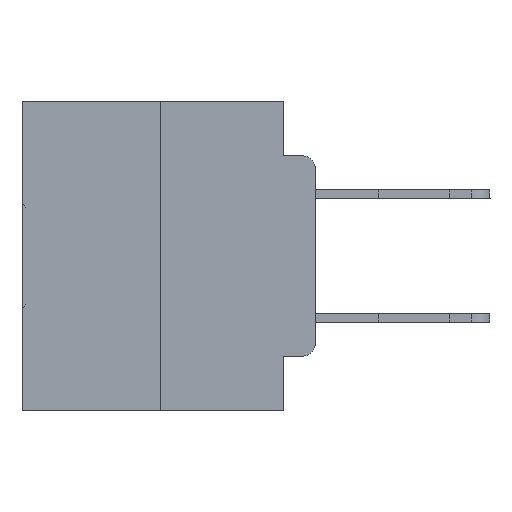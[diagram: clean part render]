
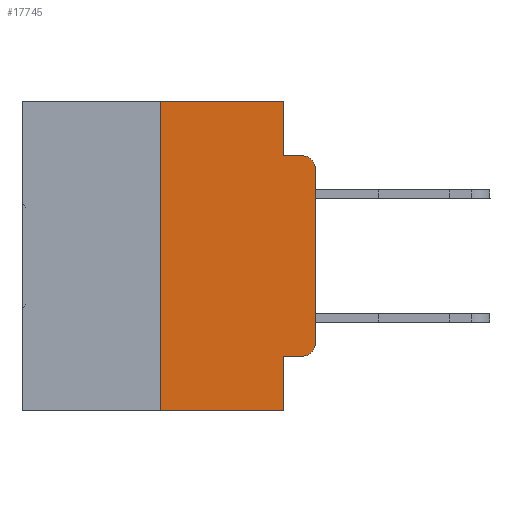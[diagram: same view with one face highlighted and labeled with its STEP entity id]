
A CAD part, left-side view. The second image highlights one B-rep face of the part: STEP entity #17745.
In plain terms, the highlighted planar face has unit normal (-1, 0, 0).
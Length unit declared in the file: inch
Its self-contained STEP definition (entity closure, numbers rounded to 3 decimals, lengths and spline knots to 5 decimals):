
#335 = ORIENTED_EDGE ( 'NONE', *, *, #4271, .F. ) ;
#445 = VECTOR ( 'NONE', #6313, 39.37008 ) ;
#823 = EDGE_CURVE ( 'NONE', #12405, #17345, #31965, .T. ) ;
#1919 = CIRCLE ( 'NONE', #31262, 0.02 ) ;
#2372 = ORIENTED_EDGE ( 'NONE', *, *, #3006, .T. ) ;
#2448 = AXIS2_PLACEMENT_3D ( 'NONE', #12802, #29903, #15337 ) ;
#2671 = ORIENTED_EDGE ( 'NONE', *, *, #28006, .F. ) ;
#3006 = EDGE_CURVE ( 'NONE', #11689, #9066, #28833, .T. ) ;
#3273 = CARTESIAN_POINT ( 'NONE',  ( 0., 0.051, 0. ) ) ;
#3551 = VECTOR ( 'NONE', #8623, 39.37008 ) ;
#3740 = CARTESIAN_POINT ( 'NONE',  ( 0., 0., 0. ) ) ;
#4138 = VERTEX_POINT ( 'NONE', #29300 ) ;
#4271 = EDGE_CURVE ( 'NONE', #17345, #9781, #13915, .T. ) ;
#4368 = ORIENTED_EDGE ( 'NONE', *, *, #29582, .F. ) ;
#5059 = CARTESIAN_POINT ( 'NONE',  ( 0., 0.051, -0.4115 ) ) ;
#6313 = DIRECTION ( 'NONE',  ( 0., 0., 1. ) ) ;
#6607 = DIRECTION ( 'NONE',  ( -1., 0., 0. ) ) ;
#7069 = CARTESIAN_POINT ( 'NONE',  ( 0., 0.473, 0. ) ) ;
#7554 = CARTESIAN_POINT ( 'NONE',  ( 0., 0.051, -0.4115 ) ) ;
#7565 = VECTOR ( 'NONE', #21828, 39.37008 ) ;
#7703 = EDGE_CURVE ( 'NONE', #4138, #9781, #1919, .T. ) ;
#8623 = DIRECTION ( 'NONE',  ( 0., 0., 1. ) ) ;
#9066 = VERTEX_POINT ( 'NONE', #27951 ) ;
#9092 = DIRECTION ( 'NONE',  ( -1., 0., 0. ) ) ;
#9589 = AXIS2_PLACEMENT_3D ( 'NONE', #23738, #9092, #26189 ) ;
#9726 = FACE_OUTER_BOUND ( 'NONE', #14275, .T. ) ;
#9781 = VERTEX_POINT ( 'NONE', #20885 ) ;
#9907 = LINE ( 'NONE', #7069, #22913 ) ;
#10166 = VECTOR ( 'NONE', #16653, 39.37008 ) ;
#11091 = EDGE_CURVE ( 'NONE', #13389, #4138, #13869, .T. ) ;
#11689 = VERTEX_POINT ( 'NONE', #30651 ) ;
#12196 = VECTOR ( 'NONE', #19856, 39.37008 ) ;
#12405 = VERTEX_POINT ( 'NONE', #23756 ) ;
#12802 = CARTESIAN_POINT ( 'NONE',  ( 0., 0.473, 0. ) ) ;
#13111 = VECTOR ( 'NONE', #23097, 39.37008 ) ;
#13389 = VERTEX_POINT ( 'NONE', #23079 ) ;
#13607 = CARTESIAN_POINT ( 'NONE',  ( 0., 0.25, 0. ) ) ;
#13869 = LINE ( 'NONE', #3740, #445 ) ;
#13915 = LINE ( 'NONE', #24008, #14637 ) ;
#14085 = VERTEX_POINT ( 'NONE', #20551 ) ;
#14275 = EDGE_LOOP ( 'NONE', ( #21618, #28159, #335, #15859, #25833, #4368, #2372, #2671, #26941, #21997 ) ) ;
#14637 = VECTOR ( 'NONE', #24073, 39.37008 ) ;
#15337 = DIRECTION ( 'NONE',  ( 0., 0., -1. ) ) ;
#15859 = ORIENTED_EDGE ( 'NONE', *, *, #823, .F. ) ;
#16653 = DIRECTION ( 'NONE',  ( 0., -1., 0. ) ) ;
#16803 = LINE ( 'NONE', #13607, #3551 ) ;
#17345 = VERTEX_POINT ( 'NONE', #18698 ) ;
#17745 = ADVANCED_FACE ( 'NONE', ( #9726 ), #22616, .F. ) ;
#18312 = VERTEX_POINT ( 'NONE', #7554 ) ;
#18698 = CARTESIAN_POINT ( 'NONE',  ( 0., 0.051, -0.0885 ) ) ;
#19856 = DIRECTION ( 'NONE',  ( 0., -1., 0. ) ) ;
#20377 = CARTESIAN_POINT ( 'NONE',  ( 0., 0.473, -0.5 ) ) ;
#20551 = CARTESIAN_POINT ( 'NONE',  ( 0., 0.02, -0.4115 ) ) ;
#20885 = CARTESIAN_POINT ( 'NONE',  ( 0., 0.02, -0.0885 ) ) ;
#21351 = CARTESIAN_POINT ( 'NONE',  ( 0., 0.02, -0.1085 ) ) ;
#21484 = EDGE_CURVE ( 'NONE', #14085, #13389, #31944, .T. ) ;
#21618 = ORIENTED_EDGE ( 'NONE', *, *, #11091, .T. ) ;
#21795 = CARTESIAN_POINT ( 'NONE',  ( 0., 0.051, 0. ) ) ;
#21828 = DIRECTION ( 'NONE',  ( 0., 0., -1. ) ) ;
#21997 = ORIENTED_EDGE ( 'NONE', *, *, #21484, .T. ) ;
#22616 = PLANE ( 'NONE',  #2448 ) ;
#22913 = VECTOR ( 'NONE', #24222, 39.37008 ) ;
#23079 = CARTESIAN_POINT ( 'NONE',  ( 0., 0., -0.3915 ) ) ;
#23097 = DIRECTION ( 'NONE',  ( 0., 0., -1. ) ) ;
#23738 = CARTESIAN_POINT ( 'NONE',  ( 0., 0.02, -0.3915 ) ) ;
#23756 = CARTESIAN_POINT ( 'NONE',  ( 0., 0.051, 0. ) ) ;
#23796 = DIRECTION ( 'NONE',  ( 0., 0., -1. ) ) ;
#24008 = CARTESIAN_POINT ( 'NONE',  ( 0., 0.051, -0.0885 ) ) ;
#24073 = DIRECTION ( 'NONE',  ( 0., -1., 0. ) ) ;
#24222 = DIRECTION ( 'NONE',  ( 0., -1., 0. ) ) ;
#24729 = EDGE_CURVE ( 'NONE', #18312, #14085, #25165, .T. ) ;
#25165 = LINE ( 'NONE', #5059, #12196 ) ;
#25833 = ORIENTED_EDGE ( 'NONE', *, *, #29809, .F. ) ;
#26075 = LINE ( 'NONE', #3273, #13111 ) ;
#26189 = DIRECTION ( 'NONE',  ( 0., 0., -1. ) ) ;
#26941 = ORIENTED_EDGE ( 'NONE', *, *, #24729, .T. ) ;
#27951 = CARTESIAN_POINT ( 'NONE',  ( 0., 0.051, -0.5 ) ) ;
#28006 = EDGE_CURVE ( 'NONE', #18312, #9066, #26075, .T. ) ;
#28148 = CARTESIAN_POINT ( 'NONE',  ( 0., 0.25, 0. ) ) ;
#28159 = ORIENTED_EDGE ( 'NONE', *, *, #7703, .T. ) ;
#28833 = LINE ( 'NONE', #20377, #10166 ) ;
#29300 = CARTESIAN_POINT ( 'NONE',  ( 0., 0., -0.1085 ) ) ;
#29582 = EDGE_CURVE ( 'NONE', #11689, #31768, #16803, .T. ) ;
#29809 = EDGE_CURVE ( 'NONE', #31768, #12405, #9907, .T. ) ;
#29903 = DIRECTION ( 'NONE',  ( 1., 0., 0. ) ) ;
#30651 = CARTESIAN_POINT ( 'NONE',  ( 0., 0.25, -0.5 ) ) ;
#31262 = AXIS2_PLACEMENT_3D ( 'NONE', #21351, #6607, #23796 ) ;
#31768 = VERTEX_POINT ( 'NONE', #28148 ) ;
#31944 = CIRCLE ( 'NONE', #9589, 0.02 ) ;
#31965 = LINE ( 'NONE', #21795, #7565 ) ;
